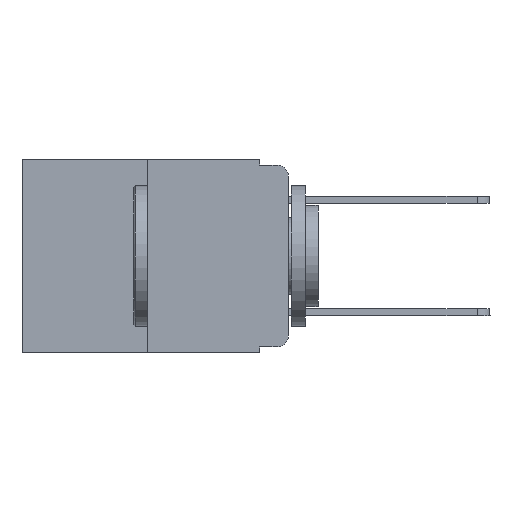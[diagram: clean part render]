
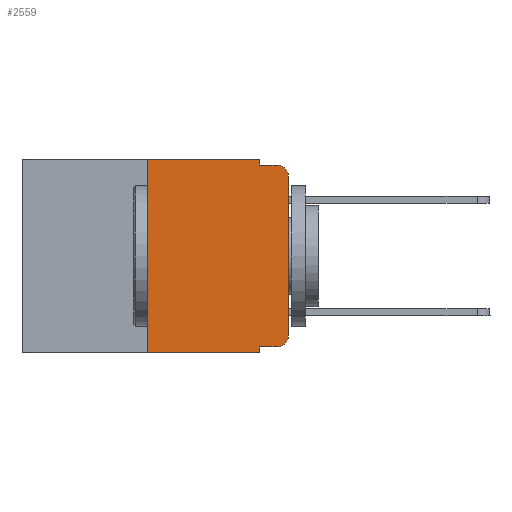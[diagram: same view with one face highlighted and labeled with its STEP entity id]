
A CAD part, left-side view. The second image highlights one B-rep face of the part: STEP entity #2559.
In plain terms, the highlighted planar face has unit normal (-1, 0, 0).
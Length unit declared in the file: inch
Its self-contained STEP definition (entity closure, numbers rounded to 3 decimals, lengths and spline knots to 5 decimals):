
#1183 = VECTOR ( 'NONE', #14076, 39.37008 ) ;
#1867 = VECTOR ( 'NONE', #13218, 39.37008 ) ;
#1935 = CARTESIAN_POINT ( 'NONE',  ( 0., 0.051, 0. ) ) ;
#2273 = CARTESIAN_POINT ( 'NONE',  ( 0., 0.051, -0.01 ) ) ;
#2467 = DIRECTION ( 'NONE',  ( 0., 0., -1. ) ) ;
#2559 = ADVANCED_FACE ( 'NONE', ( #18364 ), #16610, .F. ) ;
#2739 = ORIENTED_EDGE ( 'NONE', *, *, #5577, .T. ) ;
#2898 = AXIS2_PLACEMENT_3D ( 'NONE', #5552, #10529, #13809 ) ;
#3308 = DIRECTION ( 'NONE',  ( 0., 0., -1. ) ) ;
#3345 = VERTEX_POINT ( 'NONE', #8644 ) ;
#4245 = EDGE_CURVE ( 'NONE', #7727, #3345, #18046, .T. ) ;
#4769 = VECTOR ( 'NONE', #21774, 39.37008 ) ;
#4844 = LINE ( 'NONE', #18548, #10065 ) ;
#4949 = EDGE_CURVE ( 'NONE', #14272, #12827, #5541, .T. ) ;
#4988 = VECTOR ( 'NONE', #5760, 39.37008 ) ;
#5053 = CARTESIAN_POINT ( 'NONE',  ( 0., 0., 0. ) ) ;
#5419 = AXIS2_PLACEMENT_3D ( 'NONE', #13471, #13365, #6449 ) ;
#5465 = AXIS2_PLACEMENT_3D ( 'NONE', #14533, #11054, #2467 ) ;
#5541 = LINE ( 'NONE', #2273, #4988 ) ;
#5552 = CARTESIAN_POINT ( 'NONE',  ( 0., 0.02, -0.313 ) ) ;
#5569 = CARTESIAN_POINT ( 'NONE',  ( 0., 0.051, 0. ) ) ;
#5577 = EDGE_CURVE ( 'NONE', #9900, #12827, #15196, .T. ) ;
#5760 = DIRECTION ( 'NONE',  ( 0., -1., 0. ) ) ;
#6022 = LINE ( 'NONE', #9628, #13801 ) ;
#6050 = CARTESIAN_POINT ( 'NONE',  ( 0., 0.25, 0. ) ) ;
#6437 = ORIENTED_EDGE ( 'NONE', *, *, #17448, .F. ) ;
#6449 = DIRECTION ( 'NONE',  ( 0., 0., -1. ) ) ;
#6765 = ORIENTED_EDGE ( 'NONE', *, *, #12681, .T. ) ;
#6880 = CARTESIAN_POINT ( 'NONE',  ( 0., 0., -0.313 ) ) ;
#7160 = DIRECTION ( 'NONE',  ( 0., 0., 1. ) ) ;
#7609 = VERTEX_POINT ( 'NONE', #5569 ) ;
#7727 = VERTEX_POINT ( 'NONE', #21389 ) ;
#8258 = VERTEX_POINT ( 'NONE', #16689 ) ;
#8282 = VERTEX_POINT ( 'NONE', #13754 ) ;
#8528 = DIRECTION ( 'NONE',  ( 0., 0., 1. ) ) ;
#8644 = CARTESIAN_POINT ( 'NONE',  ( 0., 0.051, -0.343 ) ) ;
#9407 = VERTEX_POINT ( 'NONE', #6880 ) ;
#9409 = CARTESIAN_POINT ( 'NONE',  ( 0., 0.051, 0. ) ) ;
#9628 = CARTESIAN_POINT ( 'NONE',  ( 0., 0.473, -0.343 ) ) ;
#9900 = VERTEX_POINT ( 'NONE', #9940 ) ;
#9940 = CARTESIAN_POINT ( 'NONE',  ( 0., 0., -0.03 ) ) ;
#10065 = VECTOR ( 'NONE', #8528, 39.37008 ) ;
#10515 = LINE ( 'NONE', #1935, #10923 ) ;
#10529 = DIRECTION ( 'NONE',  ( -1., 0., 0. ) ) ;
#10923 = VECTOR ( 'NONE', #3308, 39.37008 ) ;
#11054 = DIRECTION ( 'NONE',  ( -1., 0., 0. ) ) ;
#11678 = EDGE_CURVE ( 'NONE', #8258, #21261, #4844, .T. ) ;
#12679 = CARTESIAN_POINT ( 'NONE',  ( 0., 0.02, -0.01 ) ) ;
#12681 = EDGE_CURVE ( 'NONE', #8282, #9407, #19160, .T. ) ;
#12731 = ORIENTED_EDGE ( 'NONE', *, *, #11678, .F. ) ;
#12827 = VERTEX_POINT ( 'NONE', #12679 ) ;
#12882 = ORIENTED_EDGE ( 'NONE', *, *, #17228, .T. ) ;
#13100 = CARTESIAN_POINT ( 'NONE',  ( 0., 0.473, 0. ) ) ;
#13218 = DIRECTION ( 'NONE',  ( 0., 0., -1. ) ) ;
#13365 = DIRECTION ( 'NONE',  ( 1., 0., 0. ) ) ;
#13471 = CARTESIAN_POINT ( 'NONE',  ( 0., 0.473, 0. ) ) ;
#13754 = CARTESIAN_POINT ( 'NONE',  ( 0., 0.02, -0.333 ) ) ;
#13801 = VECTOR ( 'NONE', #18378, 39.37008 ) ;
#13809 = DIRECTION ( 'NONE',  ( 0., 0., -1. ) ) ;
#13877 = EDGE_CURVE ( 'NONE', #9407, #9900, #20541, .T. ) ;
#13973 = EDGE_LOOP ( 'NONE', ( #17689, #2739, #15242, #6437, #17771, #12731, #16017, #14440, #12882, #6765 ) ) ;
#14076 = DIRECTION ( 'NONE',  ( 0., -1., 0. ) ) ;
#14189 = CARTESIAN_POINT ( 'NONE',  ( 0., 0.051, -0.333 ) ) ;
#14272 = VERTEX_POINT ( 'NONE', #15074 ) ;
#14407 = VECTOR ( 'NONE', #7160, 39.37008 ) ;
#14440 = ORIENTED_EDGE ( 'NONE', *, *, #4245, .F. ) ;
#14533 = CARTESIAN_POINT ( 'NONE',  ( 0., 0.02, -0.03 ) ) ;
#14755 = LINE ( 'NONE', #13100, #4769 ) ;
#15074 = CARTESIAN_POINT ( 'NONE',  ( 0., 0.051, -0.01 ) ) ;
#15196 = CIRCLE ( 'NONE', #5465, 0.02 ) ;
#15242 = ORIENTED_EDGE ( 'NONE', *, *, #4949, .F. ) ;
#16017 = ORIENTED_EDGE ( 'NONE', *, *, #20386, .T. ) ;
#16610 = PLANE ( 'NONE',  #5419 ) ;
#16689 = CARTESIAN_POINT ( 'NONE',  ( 0., 0.25, -0.343 ) ) ;
#17228 = EDGE_CURVE ( 'NONE', #7727, #8282, #21196, .T. ) ;
#17448 = EDGE_CURVE ( 'NONE', #7609, #14272, #10515, .T. ) ;
#17689 = ORIENTED_EDGE ( 'NONE', *, *, #13877, .T. ) ;
#17771 = ORIENTED_EDGE ( 'NONE', *, *, #19521, .F. ) ;
#18046 = LINE ( 'NONE', #9409, #1867 ) ;
#18364 = FACE_OUTER_BOUND ( 'NONE', #13973, .T. ) ;
#18378 = DIRECTION ( 'NONE',  ( 0., -1., 0. ) ) ;
#18548 = CARTESIAN_POINT ( 'NONE',  ( 0., 0.25, 0. ) ) ;
#19160 = CIRCLE ( 'NONE', #2898, 0.02 ) ;
#19521 = EDGE_CURVE ( 'NONE', #21261, #7609, #14755, .T. ) ;
#20386 = EDGE_CURVE ( 'NONE', #8258, #3345, #6022, .T. ) ;
#20541 = LINE ( 'NONE', #5053, #14407 ) ;
#21196 = LINE ( 'NONE', #14189, #1183 ) ;
#21261 = VERTEX_POINT ( 'NONE', #6050 ) ;
#21389 = CARTESIAN_POINT ( 'NONE',  ( 0., 0.051, -0.333 ) ) ;
#21774 = DIRECTION ( 'NONE',  ( 0., -1., 0. ) ) ;
